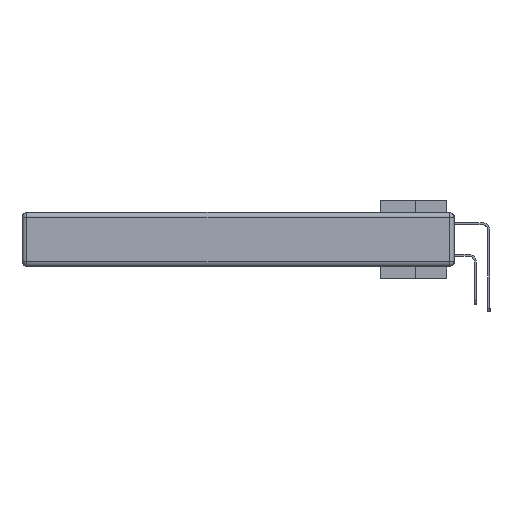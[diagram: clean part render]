
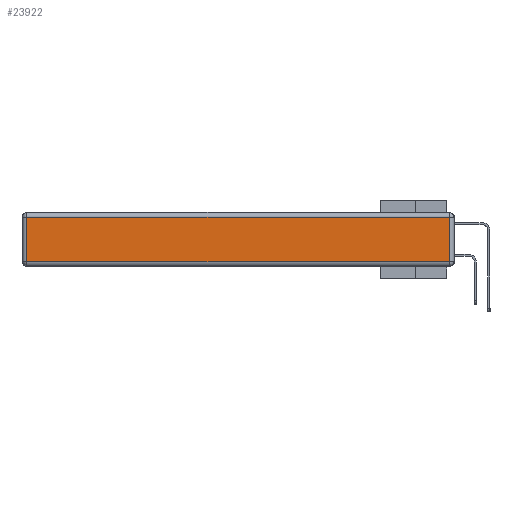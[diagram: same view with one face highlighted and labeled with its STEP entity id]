
A CAD part, left-side view. The second image highlights one B-rep face of the part: STEP entity #23922.
In plain terms, the highlighted planar face has unit normal (-1, 0, 0).
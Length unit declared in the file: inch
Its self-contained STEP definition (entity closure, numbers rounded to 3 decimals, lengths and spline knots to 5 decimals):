
#908 = DIRECTION ( 'NONE',  ( 0., -1., 0. ) ) ;
#3270 = DIRECTION ( 'NONE',  ( 0., 0., 1. ) ) ;
#3321 = VERTEX_POINT ( 'NONE', #20100 ) ;
#4026 = CARTESIAN_POINT ( 'NONE',  ( 0., 2.75, -0.03 ) ) ;
#5332 = EDGE_CURVE ( 'NONE', #11234, #3321, #9087, .T. ) ;
#7245 = VERTEX_POINT ( 'NONE', #9395 ) ;
#7806 = CARTESIAN_POINT ( 'NONE',  ( 0., 0., -0.343 ) ) ;
#7859 = CARTESIAN_POINT ( 'NONE',  ( 0., 2.72, -0.343 ) ) ;
#8380 = DIRECTION ( 'NONE',  ( 0., 0., -1. ) ) ;
#9087 = LINE ( 'NONE', #4026, #32480 ) ;
#9395 = CARTESIAN_POINT ( 'NONE',  ( 0., 0.03, -0.313 ) ) ;
#9571 = VERTEX_POINT ( 'NONE', #27191 ) ;
#9677 = EDGE_CURVE ( 'NONE', #3321, #9571, #31924, .T. ) ;
#10275 = FACE_OUTER_BOUND ( 'NONE', #16955, .T. ) ;
#11185 = VECTOR ( 'NONE', #8380, 39.37008 ) ;
#11234 = VERTEX_POINT ( 'NONE', #15098 ) ;
#14313 = AXIS2_PLACEMENT_3D ( 'NONE', #7806, #29233, #3270 ) ;
#14352 = VECTOR ( 'NONE', #29977, 39.37008 ) ;
#14756 = LINE ( 'NONE', #22513, #14989 ) ;
#14989 = VECTOR ( 'NONE', #908, 39.37008 ) ;
#15098 = CARTESIAN_POINT ( 'NONE',  ( 0., 0.03, -0.03 ) ) ;
#16955 = EDGE_LOOP ( 'NONE', ( #27681, #20630, #23317, #28786 ) ) ;
#19481 = DIRECTION ( 'NONE',  ( 0., 1., 0. ) ) ;
#20100 = CARTESIAN_POINT ( 'NONE',  ( 0., 2.72, -0.03 ) ) ;
#20609 = EDGE_CURVE ( 'NONE', #9571, #7245, #14756, .T. ) ;
#20630 = ORIENTED_EDGE ( 'NONE', *, *, #27212, .T. ) ;
#21929 = CARTESIAN_POINT ( 'NONE',  ( 0., 0.03, -0.343 ) ) ;
#22513 = CARTESIAN_POINT ( 'NONE',  ( 0., 0., -0.313 ) ) ;
#23317 = ORIENTED_EDGE ( 'NONE', *, *, #5332, .T. ) ;
#23922 = ADVANCED_FACE ( 'NONE', ( #10275 ), #31700, .T. ) ;
#24377 = LINE ( 'NONE', #21929, #14352 ) ;
#27191 = CARTESIAN_POINT ( 'NONE',  ( 0., 2.72, -0.313 ) ) ;
#27212 = EDGE_CURVE ( 'NONE', #7245, #11234, #24377, .T. ) ;
#27681 = ORIENTED_EDGE ( 'NONE', *, *, #20609, .T. ) ;
#28786 = ORIENTED_EDGE ( 'NONE', *, *, #9677, .T. ) ;
#29233 = DIRECTION ( 'NONE',  ( -1., 0., 0. ) ) ;
#29977 = DIRECTION ( 'NONE',  ( 0., 0., 1. ) ) ;
#31700 = PLANE ( 'NONE',  #14313 ) ;
#31924 = LINE ( 'NONE', #7859, #11185 ) ;
#32480 = VECTOR ( 'NONE', #19481, 39.37008 ) ;
